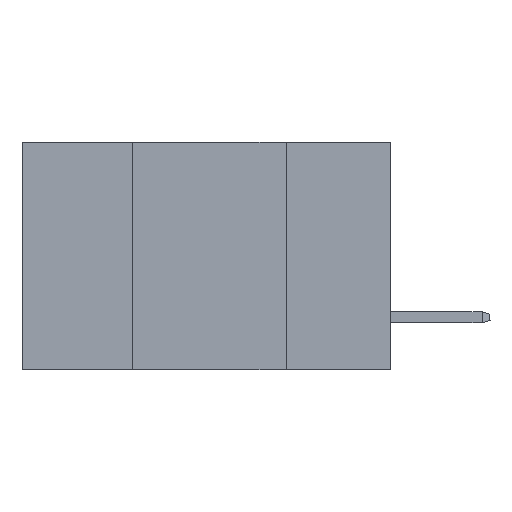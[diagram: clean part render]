
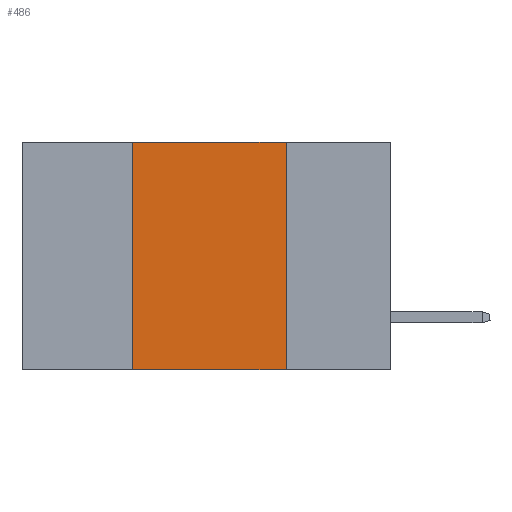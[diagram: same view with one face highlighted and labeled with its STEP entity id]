
A CAD part, left-side view. The second image highlights one B-rep face of the part: STEP entity #486.
In plain terms, the highlighted planar face has unit normal (-1, 0, 0).
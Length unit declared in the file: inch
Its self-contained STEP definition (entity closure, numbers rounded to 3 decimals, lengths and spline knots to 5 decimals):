
#486 = ADVANCED_FACE ( 'NONE', ( #27283 ), #40469, .F. ) ;
#777 = CARTESIAN_POINT ( 'NONE',  ( 0., 0.6, 0. ) ) ;
#5188 = ORIENTED_EDGE ( 'NONE', *, *, #7585, .F. ) ;
#7364 = DIRECTION ( 'NONE',  ( 0., 0., 1. ) ) ;
#7585 = EDGE_CURVE ( 'NONE', #24763, #14743, #35220, .T. ) ;
#8612 = VECTOR ( 'NONE', #7364, 39.37008 ) ;
#11244 = DIRECTION ( 'NONE',  ( 0., -1., 0. ) ) ;
#11298 = ORIENTED_EDGE ( 'NONE', *, *, #32351, .T. ) ;
#13137 = EDGE_LOOP ( 'NONE', ( #5188, #21027, #40256, #11298 ) ) ;
#14140 = LINE ( 'NONE', #28297, #29977 ) ;
#14743 = VERTEX_POINT ( 'NONE', #25632 ) ;
#17418 = VERTEX_POINT ( 'NONE', #41643 ) ;
#17468 = LINE ( 'NONE', #27512, #8612 ) ;
#18389 = EDGE_CURVE ( 'NONE', #34468, #24763, #30981, .T. ) ;
#18556 = CARTESIAN_POINT ( 'NONE',  ( 0., 0.17, 0. ) ) ;
#18694 = CARTESIAN_POINT ( 'NONE',  ( 0., 0.17, 0. ) ) ;
#21027 = ORIENTED_EDGE ( 'NONE', *, *, #18389, .F. ) ;
#22103 = DIRECTION ( 'NONE',  ( 0., 0., -1. ) ) ;
#24129 = AXIS2_PLACEMENT_3D ( 'NONE', #777, #27177, #40608 ) ;
#24763 = VERTEX_POINT ( 'NONE', #18694 ) ;
#25632 = CARTESIAN_POINT ( 'NONE',  ( 0., 0.17, -0.37 ) ) ;
#27177 = DIRECTION ( 'NONE',  ( 1., 0., 0. ) ) ;
#27283 = FACE_OUTER_BOUND ( 'NONE', #13137, .T. ) ;
#27512 = CARTESIAN_POINT ( 'NONE',  ( 0., 0.42, 0. ) ) ;
#28297 = CARTESIAN_POINT ( 'NONE',  ( 0., 0.6, -0.37 ) ) ;
#28403 = VECTOR ( 'NONE', #11244, 39.37008 ) ;
#29977 = VECTOR ( 'NONE', #31941, 39.37008 ) ;
#30981 = LINE ( 'NONE', #37072, #28403 ) ;
#31589 = CARTESIAN_POINT ( 'NONE',  ( 0., 0.42, 0. ) ) ;
#31941 = DIRECTION ( 'NONE',  ( 0., -1., 0. ) ) ;
#32351 = EDGE_CURVE ( 'NONE', #17418, #14743, #14140, .T. ) ;
#34468 = VERTEX_POINT ( 'NONE', #31589 ) ;
#35220 = LINE ( 'NONE', #18556, #36783 ) ;
#36161 = EDGE_CURVE ( 'NONE', #17418, #34468, #17468, .T. ) ;
#36783 = VECTOR ( 'NONE', #22103, 39.37008 ) ;
#37072 = CARTESIAN_POINT ( 'NONE',  ( 0., 0.6, 0. ) ) ;
#40256 = ORIENTED_EDGE ( 'NONE', *, *, #36161, .F. ) ;
#40469 = PLANE ( 'NONE',  #24129 ) ;
#40608 = DIRECTION ( 'NONE',  ( 0., 0., -1. ) ) ;
#41643 = CARTESIAN_POINT ( 'NONE',  ( 0., 0.42, -0.37 ) ) ;
